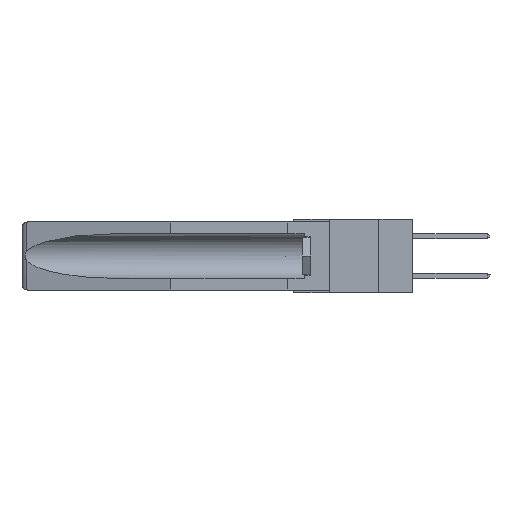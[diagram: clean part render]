
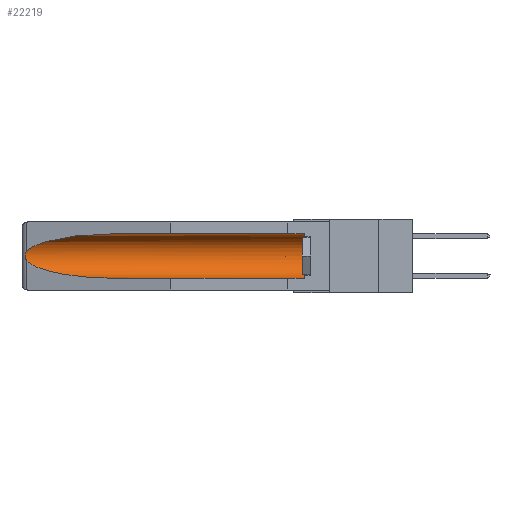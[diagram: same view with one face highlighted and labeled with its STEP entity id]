
A CAD part, left-side view. The second image highlights one B-rep face of the part: STEP entity #22219.
In plain terms, the highlighted cylindrical face has radius 2.857 mm (diameter 5.715 mm), a partial arc.
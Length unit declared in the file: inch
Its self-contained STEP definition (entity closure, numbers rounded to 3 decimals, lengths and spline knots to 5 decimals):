
#664 = CARTESIAN_POINT ( 'NONE',  ( 0.26537, 1.52718, -0.19328 ) ) ;
#990 = CARTESIAN_POINT ( 'NONE',  ( 0.155, -0.30754, -0.1715 ) ) ;
#1422 = VERTEX_POINT ( 'NONE', #26427 ) ;
#1553 = DIRECTION ( 'NONE',  ( 0., 1., 0. ) ) ;
#2394 = DIRECTION ( 'NONE',  ( 0., 0., 1. ) ) ;
#3025 = CARTESIAN_POINT ( 'NONE',  ( 0.21114, 1.30732, -0.059 ) ) ;
#4335 =( BOUNDED_CURVE ( )  B_SPLINE_CURVE ( 3, ( #664, #25323, #13942, #5883 ),
 .UNSPECIFIED., .F., .F. ) 
 B_SPLINE_CURVE_WITH_KNOTS ( ( 4, 4 ),
 ( 0.1948, 1.5708 ),
 .UNSPECIFIED. ) 
 CURVE ( )  GEOMETRIC_REPRESENTATION_ITEM ( )  RATIONAL_B_SPLINE_CURVE ( ( 1., 0.848, 0.848, 1. ) ) 
 REPRESENTATION_ITEM ( '' )  );
#4479 = CARTESIAN_POINT ( 'NONE',  ( 0.26597, 1.52961, -0.15275 ) ) ;
#4543 =( BOUNDED_CURVE ( )  B_SPLINE_CURVE ( 3, ( #27212, #3025, #21986, #27569 ),
 .UNSPECIFIED., .F., .F. ) 
 B_SPLINE_CURVE_WITH_KNOTS ( ( 4, 4 ),
 ( 4.71239, 6.08839 ),
 .UNSPECIFIED. ) 
 CURVE ( )  GEOMETRIC_REPRESENTATION_ITEM ( )  RATIONAL_B_SPLINE_CURVE ( ( 1., 0.848, 0.848, 1. ) ) 
 REPRESENTATION_ITEM ( '' )  );
#4607 = CARTESIAN_POINT ( 'NONE',  ( 0.26597, 1.5296, -0.19026 ) ) ;
#4689 = EDGE_LOOP ( 'NONE', ( #10780, #32696, #13397, #33407, #27395, #9490 ) ) ;
#5007 = CARTESIAN_POINT ( 'NONE',  ( 0.155, 0.126, -0.1715 ) ) ;
#5715 = CARTESIAN_POINT ( 'NONE',  ( 0.155, 1.07973, -0.059 ) ) ;
#5883 = CARTESIAN_POINT ( 'NONE',  ( 0.155, 1.07973, -0.284 ) ) ;
#6129 = EDGE_CURVE ( 'NONE', #13201, #16019, #11714, .T. ) ;
#6298 = CARTESIAN_POINT ( 'NONE',  ( 0.26537, 1.52718, -0.19328 ) ) ;
#7805 = CARTESIAN_POINT ( 'NONE',  ( 0.155, -0.30754, -0.284 ) ) ;
#9253 = CARTESIAN_POINT ( 'NONE',  ( 0.155, -0.30754, -0.059 ) ) ;
#9490 = ORIENTED_EDGE ( 'NONE', *, *, #31637, .T. ) ;
#10106 = EDGE_CURVE ( 'NONE', #13035, #20451, #15183, .T. ) ;
#10780 = ORIENTED_EDGE ( 'NONE', *, *, #14625, .T. ) ;
#11344 = CYLINDRICAL_SURFACE ( 'NONE', #33131, 0.1125 ) ;
#11714 = B_SPLINE_CURVE_WITH_KNOTS ( 'NONE', 3,
 ( #17880, #4479, #26047, #18114, #28807, #34280, #12535, #15363, #4607, #34152 ),
 .UNSPECIFIED., .F., .F.,
 ( 4, 2, 2, 2, 4 ),
 ( 0., 0.00029, 0.00058, 0.00087, 0.00117 ),
 .UNSPECIFIED. ) ;
#12535 = CARTESIAN_POINT ( 'NONE',  ( 0.2673, 1.53269, -0.17917 ) ) ;
#12603 = EDGE_CURVE ( 'NONE', #16019, #1422, #4335, .T. ) ;
#13035 = VERTEX_POINT ( 'NONE', #14673 ) ;
#13201 = VERTEX_POINT ( 'NONE', #28686 ) ;
#13397 = ORIENTED_EDGE ( 'NONE', *, *, #12603, .T. ) ;
#13407 = DIRECTION ( 'NONE',  ( 0., -1., 0. ) ) ;
#13942 = CARTESIAN_POINT ( 'NONE',  ( 0.21114, 1.30732, -0.284 ) ) ;
#14048 = VECTOR ( 'NONE', #1553, 39.37008 ) ;
#14625 = EDGE_CURVE ( 'NONE', #18017, #13201, #4543, .T. ) ;
#14673 = CARTESIAN_POINT ( 'NONE',  ( 0.155, 0.126, -0.284 ) ) ;
#15183 = CIRCLE ( 'NONE', #21416, 0.1125 ) ;
#15307 = LINE ( 'NONE', #9253, #14048 ) ;
#15363 = CARTESIAN_POINT ( 'NONE',  ( 0.26655, 1.53094, -0.18657 ) ) ;
#16019 = VERTEX_POINT ( 'NONE', #6298 ) ;
#16850 = FACE_OUTER_BOUND ( 'NONE', #4689, .T. ) ;
#17880 = CARTESIAN_POINT ( 'NONE',  ( 0.26537, 1.52718, -0.14972 ) ) ;
#18017 = VERTEX_POINT ( 'NONE', #5715 ) ;
#18114 = CARTESIAN_POINT ( 'NONE',  ( 0.2673, 1.5327, -0.16383 ) ) ;
#19569 = VECTOR ( 'NONE', #32131, 39.37008 ) ;
#20451 = VERTEX_POINT ( 'NONE', #32258 ) ;
#21416 = AXIS2_PLACEMENT_3D ( 'NONE', #5007, #13407, #2394 ) ;
#21986 = CARTESIAN_POINT ( 'NONE',  ( 0.25451, 1.48313, -0.09465 ) ) ;
#22219 = ADVANCED_FACE ( 'NONE', ( #16850 ), #11344, .F. ) ;
#22815 = DIRECTION ( 'NONE',  ( 0., 1., 0. ) ) ;
#25323 = CARTESIAN_POINT ( 'NONE',  ( 0.25451, 1.48313, -0.24835 ) ) ;
#25760 = EDGE_CURVE ( 'NONE', #13035, #1422, #33575, .T. ) ;
#26047 = CARTESIAN_POINT ( 'NONE',  ( 0.26654, 1.53092, -0.15636 ) ) ;
#26427 = CARTESIAN_POINT ( 'NONE',  ( 0.155, 1.07973, -0.284 ) ) ;
#27212 = CARTESIAN_POINT ( 'NONE',  ( 0.155, 1.07973, -0.059 ) ) ;
#27395 = ORIENTED_EDGE ( 'NONE', *, *, #10106, .T. ) ;
#27569 = CARTESIAN_POINT ( 'NONE',  ( 0.26537, 1.52718, -0.14972 ) ) ;
#28686 = CARTESIAN_POINT ( 'NONE',  ( 0.26537, 1.52718, -0.14972 ) ) ;
#28807 = CARTESIAN_POINT ( 'NONE',  ( 0.2675, 1.53308, -0.16763 ) ) ;
#31637 = EDGE_CURVE ( 'NONE', #20451, #18017, #15307, .T. ) ;
#32131 = DIRECTION ( 'NONE',  ( 0., 1., 0. ) ) ;
#32258 = CARTESIAN_POINT ( 'NONE',  ( 0.155, 0.126, -0.059 ) ) ;
#32696 = ORIENTED_EDGE ( 'NONE', *, *, #6129, .T. ) ;
#33131 = AXIS2_PLACEMENT_3D ( 'NONE', #990, #22815, #33765 ) ;
#33407 = ORIENTED_EDGE ( 'NONE', *, *, #25760, .F. ) ;
#33575 = LINE ( 'NONE', #7805, #19569 ) ;
#33765 = DIRECTION ( 'NONE',  ( 0., 0., 1. ) ) ;
#34152 = CARTESIAN_POINT ( 'NONE',  ( 0.26537, 1.52718, -0.19328 ) ) ;
#34280 = CARTESIAN_POINT ( 'NONE',  ( 0.2675, 1.53308, -0.17534 ) ) ;
